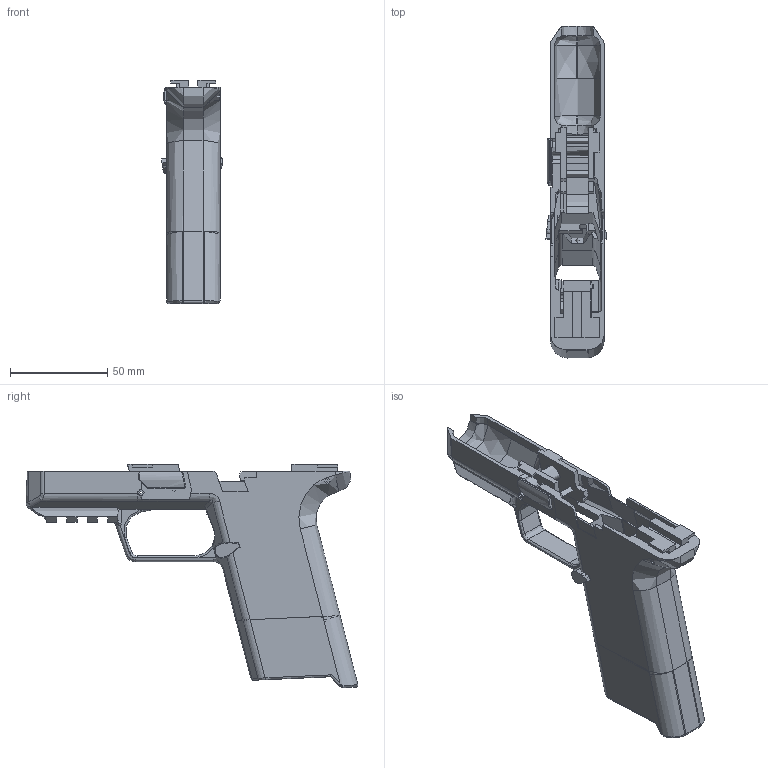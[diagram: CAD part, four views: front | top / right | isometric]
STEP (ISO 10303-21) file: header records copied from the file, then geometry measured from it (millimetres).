
FILE_DESCRIPTION(/* description */ (''),/* implementation_level */ '2;1');
FILE_NAME(/* name */ 'M&P 9 Assembly + Picatinny - Compact Length Slide.step',/* time_stamp */ '2021-11-02T07:27:17-04:00',/* author */ (''),/* organization */ (''),/* preprocessor_version */ 'ST-DEVELOPER v18.1',/* originating_system */ 'Autodesk Translation Framework v10.10.0.1391',/* authorisation */ '');
FILE_SCHEMA (('AUTOMOTIVE_DESIGN { 1 0 10303 214 3 1 1 }'));
Length unit declared in the file: millimetre
Products named in the file (13): M&P 9 Compact Length Slide - Picatinny; M&P 9 Reference v94; Rear Fire Control Group Pin; Front Locking Block Group Pin; Trigger Pin; Locking Block; Disassembly Lug; Rear Fire Control Group; Frame; Fitment Section; Nose; Magazine Release Button; Full-Size Magwell Body
Assembly tree (12 placements, depth 5):
  M&P 9 Compact Length Slide - Picatinny
    M&P 9 Reference v94
      Rear Fire Control Group Pin
      Front Locking Block Group Pin
      Trigger Pin
      Locking Block
      Disassembly Lug
      Rear Fire Control Group
      Frame
        Fitment Section
          Nose
        Magazine Release Button
        Full-Size Magwell Body
Bounding box: 30.85 x 170.13 x 114.63 mm (x, y, z)
Volume: 103010.6 mm3; surface area: 56424.9 mm2
Topology: 11 solids, 11 shells, 642 faces, 1757 edges, 1123 vertices
Faces by surface type: plane 344, cylinder 194, bspline 82, torus 17, sphere 4, cone 1
Full cylindrical faces by diameter (mm): 1.35 x2, 2 x3, 3.15 x2, 3.18 x3, 3.2 x2, 3.361 x2, 3.5 x1, 3.55 x4, 4.7 x1, 6.3 x1, 7.7 x1, 8.8 x1, 9 x2
Entity records: 23562 total; most frequent: CARTESIAN_POINT 6992, ORIENTED_EDGE 3506, DIRECTION 3265, EDGE_CURVE 1753, VERTEX_POINT 1123, LINE 1105, VECTOR 1105, AXIS2_PLACEMENT_3D 1080
